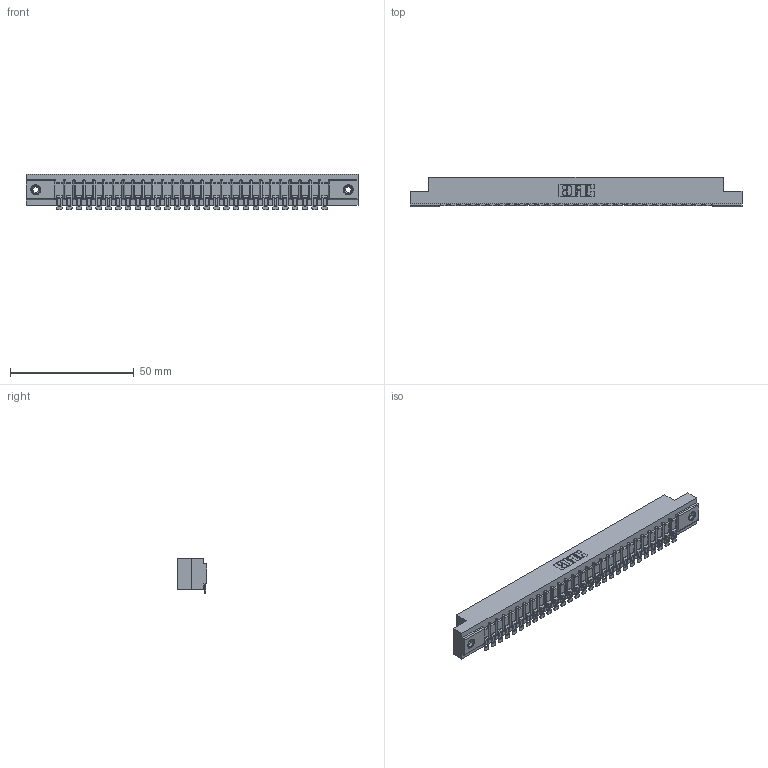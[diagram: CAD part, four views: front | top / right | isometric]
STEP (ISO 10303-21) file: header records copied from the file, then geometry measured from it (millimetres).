
FILE_DESCRIPTION (( 'STEP AP203' ), '1' );
FILE_NAME ('307-028-554-108.STEP', '2018-08-04T16:31:27', ( '' ), ( '' ), 'SwSTEP 2.0', 'SolidWorks 2016', '' );
FILE_SCHEMA (( 'CONFIG_CONTROL_DESIGN' ));
Length unit declared in the file: inch
Products named in the file (4): 307 Part_.156 Dia Mounting Holes; 307-290-002_554; 345-250-001_345-250-003-102; 307-028-554-108
Assembly tree (31 placements, depth 2):
  307-028-554-108
    307 Part_.156 Dia Mounting Holes
    307-290-002_554  x28
    345-250-001_345-250-003-102  x2
Bounding box: 133.96 x 12.01 x 14.52 mm (x, y, z)
Volume: 14234.5 mm3; surface area: 17718.9 mm2
Topology: 31 solids, 31 shells, 2475 faces, 7543 edges, 4942 vertices
Faces by surface type: plane 1390, cylinder 1011, sphere 58, cone 12, torus 4
Entity records: 27880 total; most frequent: CARTESIAN_POINT 4681, ORIENTED_EDGE 4664, DIRECTION 4570, EDGE_CURVE 2332, LINE 1772, VECTOR 1772, VERTEX_POINT 1510, AXIS2_PLACEMENT_3D 1399
